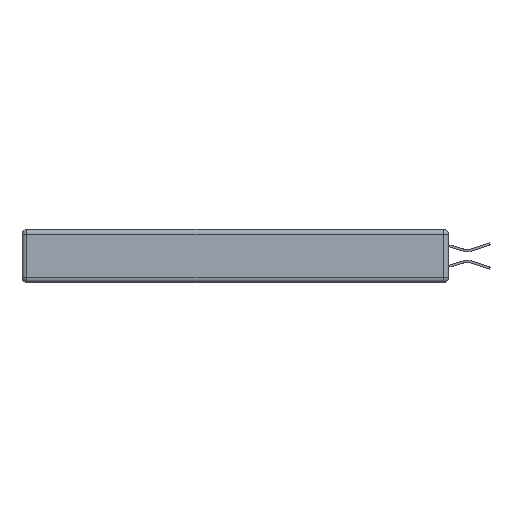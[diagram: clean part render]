
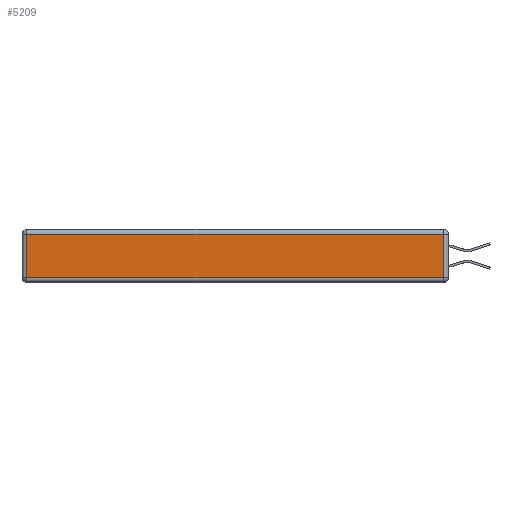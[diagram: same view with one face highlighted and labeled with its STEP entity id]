
A CAD part, left-side view. The second image highlights one B-rep face of the part: STEP entity #5209.
In plain terms, the highlighted planar face has unit normal (-1, 0, 0).
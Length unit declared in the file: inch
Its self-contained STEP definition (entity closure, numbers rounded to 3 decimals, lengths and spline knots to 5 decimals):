
#92 = CARTESIAN_POINT ( 'NONE',  ( 0., 0.03, -0.343 ) ) ;
#572 = CARTESIAN_POINT ( 'NONE',  ( 0., 0.03, -0.03 ) ) ;
#2632 = CARTESIAN_POINT ( 'NONE',  ( 0., 0., -0.313 ) ) ;
#2683 = LINE ( 'NONE', #2632, #6585 ) ;
#3560 = ORIENTED_EDGE ( 'NONE', *, *, #7976, .T. ) ;
#4106 = VERTEX_POINT ( 'NONE', #13534 ) ;
#4251 = AXIS2_PLACEMENT_3D ( 'NONE', #15095, #8684, #6231 ) ;
#4407 = ORIENTED_EDGE ( 'NONE', *, *, #14180, .T. ) ;
#4588 = FACE_OUTER_BOUND ( 'NONE', #5215, .T. ) ;
#4769 = CARTESIAN_POINT ( 'NONE',  ( 0., 2.72, -0.343 ) ) ;
#5009 = ORIENTED_EDGE ( 'NONE', *, *, #15088, .T. ) ;
#5209 = ADVANCED_FACE ( 'NONE', ( #4588 ), #13734, .T. ) ;
#5215 = EDGE_LOOP ( 'NONE', ( #11752, #5009, #4407, #3560 ) ) ;
#5220 = EDGE_CURVE ( 'NONE', #4106, #12807, #2683, .T. ) ;
#5727 = VERTEX_POINT ( 'NONE', #7419 ) ;
#5980 = DIRECTION ( 'NONE',  ( 0., 0., -1. ) ) ;
#6231 = DIRECTION ( 'NONE',  ( 0., 0., 1. ) ) ;
#6296 = CARTESIAN_POINT ( 'NONE',  ( 0., 0.03, -0.313 ) ) ;
#6585 = VECTOR ( 'NONE', #15151, 39.37008 ) ;
#6914 = VECTOR ( 'NONE', #5980, 39.37008 ) ;
#7419 = CARTESIAN_POINT ( 'NONE',  ( 0., 2.72, -0.03 ) ) ;
#7976 = EDGE_CURVE ( 'NONE', #5727, #4106, #14547, .T. ) ;
#8262 = LINE ( 'NONE', #16200, #11199 ) ;
#8684 = DIRECTION ( 'NONE',  ( -1., 0., 0. ) ) ;
#9882 = DIRECTION ( 'NONE',  ( 0., 1., 0. ) ) ;
#10367 = VERTEX_POINT ( 'NONE', #572 ) ;
#11199 = VECTOR ( 'NONE', #9882, 39.37008 ) ;
#11358 = VECTOR ( 'NONE', #12519, 39.37008 ) ;
#11569 = LINE ( 'NONE', #92, #11358 ) ;
#11752 = ORIENTED_EDGE ( 'NONE', *, *, #5220, .T. ) ;
#12519 = DIRECTION ( 'NONE',  ( 0., 0., 1. ) ) ;
#12807 = VERTEX_POINT ( 'NONE', #6296 ) ;
#13534 = CARTESIAN_POINT ( 'NONE',  ( 0., 2.72, -0.313 ) ) ;
#13734 = PLANE ( 'NONE',  #4251 ) ;
#14180 = EDGE_CURVE ( 'NONE', #10367, #5727, #8262, .T. ) ;
#14547 = LINE ( 'NONE', #4769, #6914 ) ;
#15088 = EDGE_CURVE ( 'NONE', #12807, #10367, #11569, .T. ) ;
#15095 = CARTESIAN_POINT ( 'NONE',  ( 0., 0., -0.343 ) ) ;
#15151 = DIRECTION ( 'NONE',  ( 0., -1., 0. ) ) ;
#16200 = CARTESIAN_POINT ( 'NONE',  ( 0., 2.75, -0.03 ) ) ;
